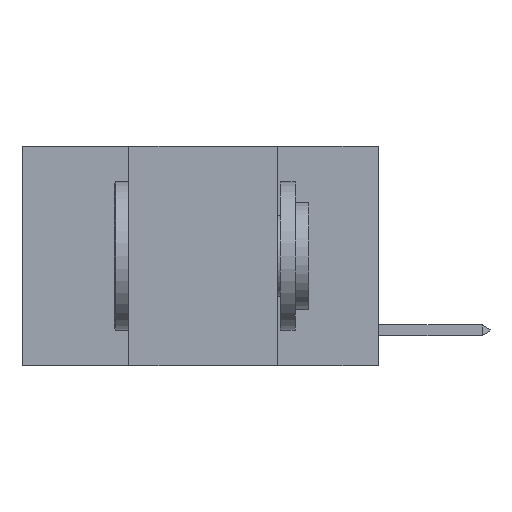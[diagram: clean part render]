
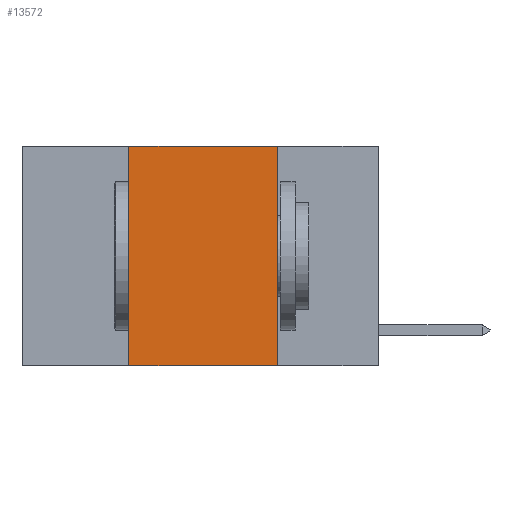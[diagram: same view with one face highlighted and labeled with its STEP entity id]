
A CAD part, left-side view. The second image highlights one B-rep face of the part: STEP entity #13572.
In plain terms, the highlighted planar face has unit normal (-1, 0, 0).
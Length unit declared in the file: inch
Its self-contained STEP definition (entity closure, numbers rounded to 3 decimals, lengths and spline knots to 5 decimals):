
#132 = CARTESIAN_POINT ( 'NONE',  ( 0., 0.42, -0.37 ) ) ;
#618 = LINE ( 'NONE', #7296, #15444 ) ;
#636 = VERTEX_POINT ( 'NONE', #132 ) ;
#1232 = CARTESIAN_POINT ( 'NONE',  ( 0., 0.6, -0.37 ) ) ;
#1280 = ORIENTED_EDGE ( 'NONE', *, *, #16186, .T. ) ;
#2554 = VERTEX_POINT ( 'NONE', #4454 ) ;
#2641 = VECTOR ( 'NONE', #7835, 39.37008 ) ;
#2935 = PLANE ( 'NONE',  #9251 ) ;
#3039 = VERTEX_POINT ( 'NONE', #16860 ) ;
#3219 = VECTOR ( 'NONE', #12998, 39.37008 ) ;
#4035 = EDGE_CURVE ( 'NONE', #636, #16474, #15686, .T. ) ;
#4093 = DIRECTION ( 'NONE',  ( 0., -1., 0. ) ) ;
#4408 = EDGE_CURVE ( 'NONE', #3039, #2554, #618, .T. ) ;
#4454 = CARTESIAN_POINT ( 'NONE',  ( 0., 0.17, -0.37 ) ) ;
#4861 = EDGE_CURVE ( 'NONE', #16474, #3039, #7692, .T. ) ;
#5461 = DIRECTION ( 'NONE',  ( 1., 0., 0. ) ) ;
#5558 = DIRECTION ( 'NONE',  ( 0., 0., -1. ) ) ;
#6359 = CARTESIAN_POINT ( 'NONE',  ( 0., 0.42, 0. ) ) ;
#6680 = FACE_OUTER_BOUND ( 'NONE', #11915, .T. ) ;
#7296 = CARTESIAN_POINT ( 'NONE',  ( 0., 0.17, 0. ) ) ;
#7469 = DIRECTION ( 'NONE',  ( 0., 0., -1. ) ) ;
#7692 = LINE ( 'NONE', #14300, #3219 ) ;
#7835 = DIRECTION ( 'NONE',  ( 0., 0., 1. ) ) ;
#8796 = VECTOR ( 'NONE', #4093, 39.37008 ) ;
#9251 = AXIS2_PLACEMENT_3D ( 'NONE', #10838, #5461, #5558 ) ;
#9385 = LINE ( 'NONE', #1232, #8796 ) ;
#9883 = ORIENTED_EDGE ( 'NONE', *, *, #4035, .F. ) ;
#10838 = CARTESIAN_POINT ( 'NONE',  ( 0., 0.6, 0. ) ) ;
#11915 = EDGE_LOOP ( 'NONE', ( #13298, #14773, #9883, #1280 ) ) ;
#12998 = DIRECTION ( 'NONE',  ( 0., -1., 0. ) ) ;
#13298 = ORIENTED_EDGE ( 'NONE', *, *, #4408, .F. ) ;
#13572 = ADVANCED_FACE ( 'NONE', ( #6680 ), #2935, .F. ) ;
#14300 = CARTESIAN_POINT ( 'NONE',  ( 0., 0.6, 0. ) ) ;
#14773 = ORIENTED_EDGE ( 'NONE', *, *, #4861, .F. ) ;
#15444 = VECTOR ( 'NONE', #7469, 39.37008 ) ;
#15686 = LINE ( 'NONE', #6359, #2641 ) ;
#16186 = EDGE_CURVE ( 'NONE', #636, #2554, #9385, .T. ) ;
#16474 = VERTEX_POINT ( 'NONE', #16639 ) ;
#16639 = CARTESIAN_POINT ( 'NONE',  ( 0., 0.42, 0. ) ) ;
#16860 = CARTESIAN_POINT ( 'NONE',  ( 0., 0.17, 0. ) ) ;
